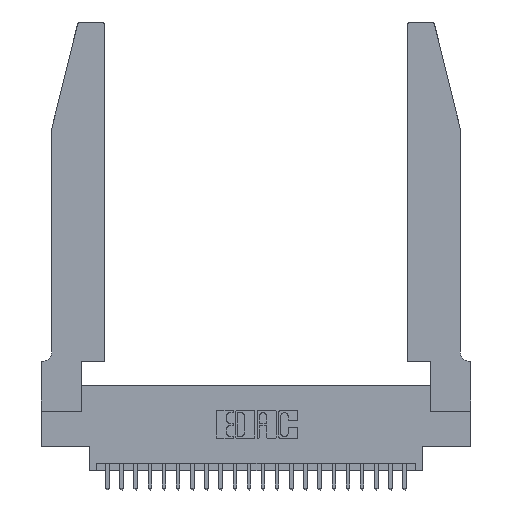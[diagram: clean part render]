
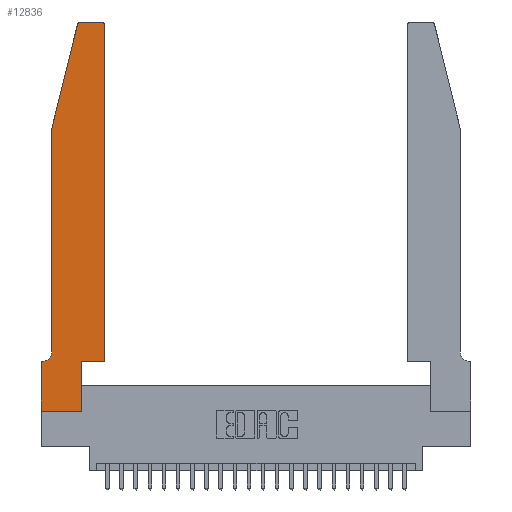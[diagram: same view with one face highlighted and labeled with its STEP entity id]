
A CAD part, top view. The second image highlights one B-rep face of the part: STEP entity #12836.
In plain terms, the highlighted planar face has unit normal (0, 0, 1).
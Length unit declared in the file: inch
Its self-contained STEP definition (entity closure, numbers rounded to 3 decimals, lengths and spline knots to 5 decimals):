
#106 = CARTESIAN_POINT ( 'NONE',  ( 0.2865, 0.35, 0.37 ) ) ;
#359 = DIRECTION ( 'NONE',  ( 0., -1., 0. ) ) ;
#419 = CARTESIAN_POINT ( 'NONE',  ( 0.25487, 2.72718, 0.37 ) ) ;
#528 = EDGE_CURVE ( 'NONE', #6647, #19696, #23572, .T. ) ;
#667 = ORIENTED_EDGE ( 'NONE', *, *, #12163, .T. ) ;
#672 = ORIENTED_EDGE ( 'NONE', *, *, #21949, .T. ) ;
#898 = CARTESIAN_POINT ( 'NONE',  ( 0.4505, 0.35, 0.37 ) ) ;
#969 = CARTESIAN_POINT ( 'NONE',  ( 0.4505, 0.35, 0.37 ) ) ;
#1197 = LINE ( 'NONE', #13166, #16021 ) ;
#1595 = DIRECTION ( 'NONE',  ( -0.239, -0.971, 0. ) ) ;
#1805 = VECTOR ( 'NONE', #3403, 39.37008 ) ;
#2559 = ORIENTED_EDGE ( 'NONE', *, *, #8524, .T. ) ;
#3403 = DIRECTION ( 'NONE',  ( 1., 0., 0. ) ) ;
#3429 = VECTOR ( 'NONE', #359, 39.37008 ) ;
#3503 = DIRECTION ( 'NONE',  ( 0., -1., 0. ) ) ;
#3582 = EDGE_CURVE ( 'NONE', #16737, #21153, #1197, .T. ) ;
#3609 = VECTOR ( 'NONE', #12420, 39.37008 ) ;
#3927 = EDGE_CURVE ( 'NONE', #23951, #21263, #18921, .T. ) ;
#3979 = EDGE_CURVE ( 'NONE', #16389, #6647, #22785, .T. ) ;
#4206 = CARTESIAN_POINT ( 'NONE',  ( 0.2605, 2.75, 0.37 ) ) ;
#4266 = FACE_OUTER_BOUND ( 'NONE', #22921, .T. ) ;
#4315 = VERTEX_POINT ( 'NONE', #19156 ) ;
#4650 = CARTESIAN_POINT ( 'NONE',  ( 0., 0.35, 0.37 ) ) ;
#4659 = VECTOR ( 'NONE', #20613, 39.37008 ) ;
#5307 = CARTESIAN_POINT ( 'NONE',  ( 0.2865, 0.35, 0.37 ) ) ;
#6086 = DIRECTION ( 'NONE',  ( 0., 0., 1. ) ) ;
#6647 = VERTEX_POINT ( 'NONE', #9167 ) ;
#6803 = ORIENTED_EDGE ( 'NONE', *, *, #17299, .T. ) ;
#6869 = EDGE_CURVE ( 'NONE', #23336, #16737, #18216, .T. ) ;
#7844 = VERTEX_POINT ( 'NONE', #15232 ) ;
#8450 = EDGE_CURVE ( 'NONE', #21263, #21018, #14268, .T. ) ;
#8524 = EDGE_CURVE ( 'NONE', #4315, #23951, #13043, .T. ) ;
#8549 = ORIENTED_EDGE ( 'NONE', *, *, #11779, .T. ) ;
#8762 = VECTOR ( 'NONE', #16206, 39.37008 ) ;
#9167 = CARTESIAN_POINT ( 'NONE',  ( 0.4505, 2.72, 0.37 ) ) ;
#9393 = CIRCLE ( 'NONE', #15454, 0.07 ) ;
#9442 = VECTOR ( 'NONE', #11001, 39.37008 ) ;
#9715 = ORIENTED_EDGE ( 'NONE', *, *, #3979, .T. ) ;
#10329 = DIRECTION ( 'NONE',  ( 0., 0., -1. ) ) ;
#10469 = DIRECTION ( 'NONE',  ( 1., 0., 0. ) ) ;
#11001 = DIRECTION ( 'NONE',  ( -1., 0., 0. ) ) ;
#11516 = LINE ( 'NONE', #14935, #1805 ) ;
#11779 = EDGE_CURVE ( 'NONE', #21018, #16389, #11516, .T. ) ;
#12163 = EDGE_CURVE ( 'NONE', #15783, #7844, #9393, .T. ) ;
#12420 = DIRECTION ( 'NONE',  ( 0., 1., 0. ) ) ;
#12836 = ADVANCED_FACE ( 'NONE', ( #4266 ), #19973, .T. ) ;
#13043 = LINE ( 'NONE', #13088, #23186 ) ;
#13088 = CARTESIAN_POINT ( 'NONE',  ( 0., 0., 0.37 ) ) ;
#13166 = CARTESIAN_POINT ( 'NONE',  ( 0.0755, 2., 0.37 ) ) ;
#13500 = ORIENTED_EDGE ( 'NONE', *, *, #3582, .T. ) ;
#14266 = DIRECTION ( 'NONE',  ( 0., 0., 1. ) ) ;
#14268 = LINE ( 'NONE', #5307, #4659 ) ;
#14555 = LINE ( 'NONE', #16701, #9442 ) ;
#14617 = CARTESIAN_POINT ( 'NONE',  ( 0.0755, 0.42, 0.37 ) ) ;
#14748 = CARTESIAN_POINT ( 'NONE',  ( 0.4205, 2.72, 0.37 ) ) ;
#14935 = CARTESIAN_POINT ( 'NONE',  ( 0.4505, 0.35, 0.37 ) ) ;
#15232 = CARTESIAN_POINT ( 'NONE',  ( 0.0055, 0.35, 0.37 ) ) ;
#15454 = AXIS2_PLACEMENT_3D ( 'NONE', #21751, #10329, #23640 ) ;
#15783 = VERTEX_POINT ( 'NONE', #14617 ) ;
#15848 = CARTESIAN_POINT ( 'NONE',  ( 0.0755, 2., 0.37 ) ) ;
#16021 = VECTOR ( 'NONE', #1595, 39.37008 ) ;
#16206 = DIRECTION ( 'NONE',  ( 1., 0., 0. ) ) ;
#16389 = VERTEX_POINT ( 'NONE', #969 ) ;
#16701 = CARTESIAN_POINT ( 'NONE',  ( 0.0755, 0.35, 0.37 ) ) ;
#16737 = VERTEX_POINT ( 'NONE', #419 ) ;
#17079 = ORIENTED_EDGE ( 'NONE', *, *, #3927, .T. ) ;
#17088 = AXIS2_PLACEMENT_3D ( 'NONE', #4650, #21890, #10469 ) ;
#17299 = EDGE_CURVE ( 'NONE', #7844, #4315, #14555, .T. ) ;
#17538 = CARTESIAN_POINT ( 'NONE',  ( 0.284, 2.72, 0.37 ) ) ;
#18216 = CIRCLE ( 'NONE', #24752, 0.03 ) ;
#18756 = LINE ( 'NONE', #23391, #3429 ) ;
#18921 = LINE ( 'NONE', #19932, #8762 ) ;
#18947 = CARTESIAN_POINT ( 'NONE',  ( 0., 0., 0.37 ) ) ;
#19110 = VECTOR ( 'NONE', #19549, 39.37008 ) ;
#19156 = CARTESIAN_POINT ( 'NONE',  ( 0., 0.35, 0.37 ) ) ;
#19432 = DIRECTION ( 'NONE',  ( 1., 0., 0. ) ) ;
#19549 = DIRECTION ( 'NONE',  ( -1., 0., 0. ) ) ;
#19581 = CARTESIAN_POINT ( 'NONE',  ( 0.2865, 0., 0.37 ) ) ;
#19696 = VERTEX_POINT ( 'NONE', #20894 ) ;
#19932 = CARTESIAN_POINT ( 'NONE',  ( 0., 0., 0.37 ) ) ;
#19973 = PLANE ( 'NONE',  #17088 ) ;
#20583 = ORIENTED_EDGE ( 'NONE', *, *, #528, .T. ) ;
#20613 = DIRECTION ( 'NONE',  ( 0., 1., 0. ) ) ;
#20894 = CARTESIAN_POINT ( 'NONE',  ( 0.4205, 2.75, 0.37 ) ) ;
#21018 = VERTEX_POINT ( 'NONE', #106 ) ;
#21153 = VERTEX_POINT ( 'NONE', #15848 ) ;
#21263 = VERTEX_POINT ( 'NONE', #19581 ) ;
#21751 = CARTESIAN_POINT ( 'NONE',  ( 0.0055, 0.42, 0.37 ) ) ;
#21890 = DIRECTION ( 'NONE',  ( 0., 0., 1. ) ) ;
#21949 = EDGE_CURVE ( 'NONE', #19696, #23336, #24733, .T. ) ;
#22377 = ORIENTED_EDGE ( 'NONE', *, *, #8450, .T. ) ;
#22773 = AXIS2_PLACEMENT_3D ( 'NONE', #14748, #14266, #24039 ) ;
#22785 = LINE ( 'NONE', #898, #3609 ) ;
#22884 = EDGE_CURVE ( 'NONE', #21153, #15783, #18756, .T. ) ;
#22921 = EDGE_LOOP ( 'NONE', ( #672, #24252, #13500, #23040, #667, #6803, #2559, #17079, #22377, #8549, #9715, #20583 ) ) ;
#23040 = ORIENTED_EDGE ( 'NONE', *, *, #22884, .T. ) ;
#23186 = VECTOR ( 'NONE', #3503, 39.37008 ) ;
#23336 = VERTEX_POINT ( 'NONE', #24686 ) ;
#23391 = CARTESIAN_POINT ( 'NONE',  ( 0.0755, 2., 0.37 ) ) ;
#23572 = CIRCLE ( 'NONE', #22773, 0.03 ) ;
#23640 = DIRECTION ( 'NONE',  ( -1., 0., 0. ) ) ;
#23951 = VERTEX_POINT ( 'NONE', #18947 ) ;
#24039 = DIRECTION ( 'NONE',  ( 1., 0., 0. ) ) ;
#24252 = ORIENTED_EDGE ( 'NONE', *, *, #6869, .T. ) ;
#24686 = CARTESIAN_POINT ( 'NONE',  ( 0.284, 2.75, 0.37 ) ) ;
#24733 = LINE ( 'NONE', #4206, #19110 ) ;
#24752 = AXIS2_PLACEMENT_3D ( 'NONE', #17538, #6086, #19432 ) ;
